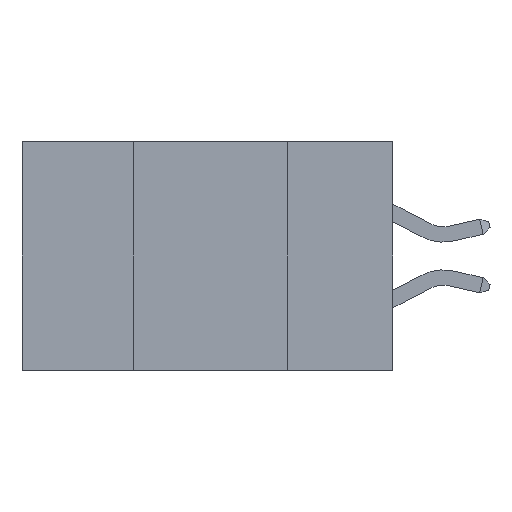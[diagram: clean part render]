
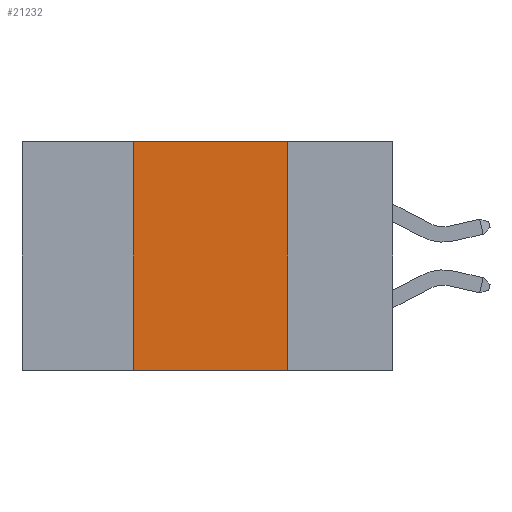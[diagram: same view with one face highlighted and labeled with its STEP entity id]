
A CAD part, left-side view. The second image highlights one B-rep face of the part: STEP entity #21232.
In plain terms, the highlighted planar face has unit normal (-1, 0, 0).
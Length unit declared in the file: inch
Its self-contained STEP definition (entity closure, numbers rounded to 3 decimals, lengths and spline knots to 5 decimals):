
#1848 = VECTOR ( 'NONE', #33416, 39.37008 ) ;
#2325 = ORIENTED_EDGE ( 'NONE', *, *, #4862, .F. ) ;
#2704 = EDGE_CURVE ( 'NONE', #12189, #2783, #27046, .T. ) ;
#2783 = VERTEX_POINT ( 'NONE', #27759 ) ;
#4054 = VERTEX_POINT ( 'NONE', #28423 ) ;
#4862 = EDGE_CURVE ( 'NONE', #12189, #28145, #7681, .T. ) ;
#6425 = PLANE ( 'NONE',  #12376 ) ;
#7681 = LINE ( 'NONE', #34948, #38850 ) ;
#8480 = VECTOR ( 'NONE', #38705, 39.37008 ) ;
#9244 = CARTESIAN_POINT ( 'NONE',  ( 0., 0.42, -0.37 ) ) ;
#9606 = DIRECTION ( 'NONE',  ( 1., 0., 0. ) ) ;
#10744 = DIRECTION ( 'NONE',  ( 0., -1., 0. ) ) ;
#11248 = EDGE_CURVE ( 'NONE', #4054, #2783, #33431, .T. ) ;
#12189 = VERTEX_POINT ( 'NONE', #9244 ) ;
#12376 = AXIS2_PLACEMENT_3D ( 'NONE', #15841, #9606, #31494 ) ;
#13293 = ORIENTED_EDGE ( 'NONE', *, *, #11248, .F. ) ;
#14776 = CARTESIAN_POINT ( 'NONE',  ( 0., 0.6, -0.37 ) ) ;
#15088 = FACE_OUTER_BOUND ( 'NONE', #21778, .T. ) ;
#15841 = CARTESIAN_POINT ( 'NONE',  ( 0., 0.6, 0. ) ) ;
#16582 = EDGE_CURVE ( 'NONE', #28145, #4054, #26915, .T. ) ;
#20200 = CARTESIAN_POINT ( 'NONE',  ( 0., 0.17, 0. ) ) ;
#21232 = ADVANCED_FACE ( 'NONE', ( #15088 ), #6425, .F. ) ;
#21778 = EDGE_LOOP ( 'NONE', ( #13293, #26537, #2325, #29443 ) ) ;
#26404 = CARTESIAN_POINT ( 'NONE',  ( 0., 0.6, 0. ) ) ;
#26537 = ORIENTED_EDGE ( 'NONE', *, *, #16582, .F. ) ;
#26915 = LINE ( 'NONE', #26404, #34132 ) ;
#27046 = LINE ( 'NONE', #14776, #1848 ) ;
#27759 = CARTESIAN_POINT ( 'NONE',  ( 0., 0.17, -0.37 ) ) ;
#28145 = VERTEX_POINT ( 'NONE', #31819 ) ;
#28423 = CARTESIAN_POINT ( 'NONE',  ( 0., 0.17, 0. ) ) ;
#29443 = ORIENTED_EDGE ( 'NONE', *, *, #2704, .T. ) ;
#31494 = DIRECTION ( 'NONE',  ( 0., 0., -1. ) ) ;
#31819 = CARTESIAN_POINT ( 'NONE',  ( 0., 0.42, 0. ) ) ;
#33416 = DIRECTION ( 'NONE',  ( 0., -1., 0. ) ) ;
#33431 = LINE ( 'NONE', #20200, #8480 ) ;
#34132 = VECTOR ( 'NONE', #10744, 39.37008 ) ;
#34948 = CARTESIAN_POINT ( 'NONE',  ( 0., 0.42, 0. ) ) ;
#38013 = DIRECTION ( 'NONE',  ( 0., 0., 1. ) ) ;
#38705 = DIRECTION ( 'NONE',  ( 0., 0., -1. ) ) ;
#38850 = VECTOR ( 'NONE', #38013, 39.37008 ) ;
